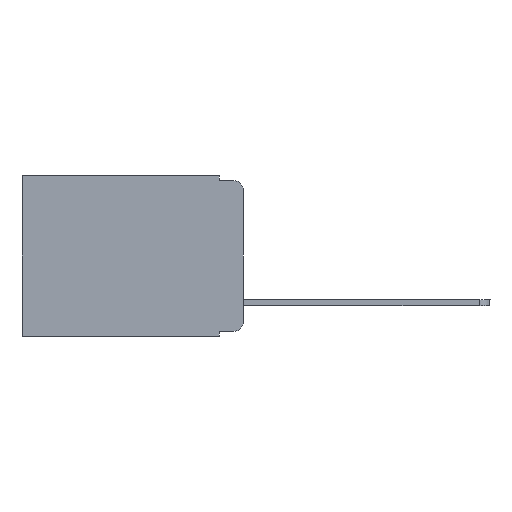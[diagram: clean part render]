
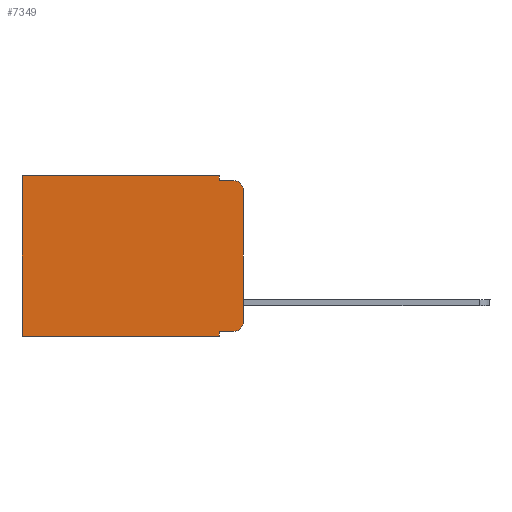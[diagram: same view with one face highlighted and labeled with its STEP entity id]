
A CAD part, left-side view. The second image highlights one B-rep face of the part: STEP entity #7349.
In plain terms, the highlighted planar face has unit normal (-1, 0, 0).
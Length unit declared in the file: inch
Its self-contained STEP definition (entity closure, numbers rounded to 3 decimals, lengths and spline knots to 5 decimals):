
#12 = EDGE_LOOP ( 'NONE', ( #2048, #13810, #19755, #18874, #17836, #16776, #1438, #20468, #11609, #22706 ) ) ;
#314 = AXIS2_PLACEMENT_3D ( 'NONE', #17217, #21081, #20713 ) ;
#598 = LINE ( 'NONE', #15646, #19737 ) ;
#1134 = VERTEX_POINT ( 'NONE', #3413 ) ;
#1438 = ORIENTED_EDGE ( 'NONE', *, *, #14756, .F. ) ;
#1525 = LINE ( 'NONE', #3345, #20152 ) ;
#1850 = VERTEX_POINT ( 'NONE', #20953 ) ;
#2048 = ORIENTED_EDGE ( 'NONE', *, *, #21662, .F. ) ;
#2523 = EDGE_CURVE ( 'NONE', #10159, #13411, #5478, .T. ) ;
#2542 = VERTEX_POINT ( 'NONE', #9267 ) ;
#3345 = CARTESIAN_POINT ( 'NONE',  ( 0.298, 0.051, 0. ) ) ;
#3413 = CARTESIAN_POINT ( 'NONE',  ( 0.298, 0.02, -0.333 ) ) ;
#3888 = DIRECTION ( 'NONE',  ( 0., 1., 0. ) ) ;
#4215 = FACE_OUTER_BOUND ( 'NONE', #12, .T. ) ;
#4271 = CARTESIAN_POINT ( 'NONE',  ( 0.298, 0., -0.03 ) ) ;
#4284 = DIRECTION ( 'NONE',  ( 0., -1., 0. ) ) ;
#4562 = DIRECTION ( 'NONE',  ( 0., 0., -1. ) ) ;
#5035 = DIRECTION ( 'NONE',  ( 0., 0., -1. ) ) ;
#5478 = LINE ( 'NONE', #5716, #11125 ) ;
#5716 = CARTESIAN_POINT ( 'NONE',  ( 0.298, 0., 0. ) ) ;
#5770 = VECTOR ( 'NONE', #23437, 39.37008 ) ;
#6905 = CARTESIAN_POINT ( 'NONE',  ( 0.298, 0.051, -0.01 ) ) ;
#7349 = ADVANCED_FACE ( 'NONE', ( #4215 ), #13361, .F. ) ;
#7800 = EDGE_CURVE ( 'NONE', #9199, #1134, #7839, .T. ) ;
#7839 = LINE ( 'NONE', #19101, #15271 ) ;
#8547 = CARTESIAN_POINT ( 'NONE',  ( 0.298, 0.02, -0.03 ) ) ;
#8747 = CARTESIAN_POINT ( 'NONE',  ( 0.298, 0.473, -0.343 ) ) ;
#8871 = VERTEX_POINT ( 'NONE', #16335 ) ;
#9199 = VERTEX_POINT ( 'NONE', #14371 ) ;
#9267 = CARTESIAN_POINT ( 'NONE',  ( 0.298, 0.051, -0.343 ) ) ;
#9456 = CARTESIAN_POINT ( 'NONE',  ( 0.298, 0.051, 0. ) ) ;
#10115 = EDGE_CURVE ( 'NONE', #1850, #12892, #16125, .T. ) ;
#10159 = VERTEX_POINT ( 'NONE', #9456 ) ;
#10241 = LINE ( 'NONE', #22938, #11379 ) ;
#10627 = DIRECTION ( 'NONE',  ( -1., 0., 0. ) ) ;
#10691 = DIRECTION ( 'NONE',  ( -1., 0., 0. ) ) ;
#11125 = VECTOR ( 'NONE', #3888, 39.37008 ) ;
#11379 = VECTOR ( 'NONE', #14103, 39.37008 ) ;
#11609 = ORIENTED_EDGE ( 'NONE', *, *, #7800, .T. ) ;
#11741 = AXIS2_PLACEMENT_3D ( 'NONE', #8547, #10627, #21252 ) ;
#12623 = DIRECTION ( 'NONE',  ( 0., -1., 0. ) ) ;
#12730 = VECTOR ( 'NONE', #12623, 39.37008 ) ;
#12798 = VECTOR ( 'NONE', #21095, 39.37008 ) ;
#12892 = VERTEX_POINT ( 'NONE', #22839 ) ;
#12999 = VERTEX_POINT ( 'NONE', #4271 ) ;
#13361 = PLANE ( 'NONE',  #314 ) ;
#13411 = VERTEX_POINT ( 'NONE', #20738 ) ;
#13734 = LINE ( 'NONE', #19397, #12798 ) ;
#13810 = ORIENTED_EDGE ( 'NONE', *, *, #14302, .T. ) ;
#14103 = DIRECTION ( 'NONE',  ( 0., 1., 0. ) ) ;
#14302 = EDGE_CURVE ( 'NONE', #12999, #12892, #22151, .T. ) ;
#14371 = CARTESIAN_POINT ( 'NONE',  ( 0.298, 0.051, -0.333 ) ) ;
#14756 = EDGE_CURVE ( 'NONE', #2542, #14995, #10241, .T. ) ;
#14881 = AXIS2_PLACEMENT_3D ( 'NONE', #19860, #10691, #18048 ) ;
#14995 = VERTEX_POINT ( 'NONE', #8747 ) ;
#15271 = VECTOR ( 'NONE', #4284, 39.37008 ) ;
#15646 = CARTESIAN_POINT ( 'NONE',  ( 0.298, 0.051, 0. ) ) ;
#15832 = LINE ( 'NONE', #17524, #5770 ) ;
#16125 = LINE ( 'NONE', #6905, #12730 ) ;
#16335 = CARTESIAN_POINT ( 'NONE',  ( 0.298, 0., -0.313 ) ) ;
#16776 = ORIENTED_EDGE ( 'NONE', *, *, #20930, .T. ) ;
#17217 = CARTESIAN_POINT ( 'NONE',  ( 0.298, 0., 0. ) ) ;
#17289 = EDGE_CURVE ( 'NONE', #1134, #8871, #18358, .T. ) ;
#17524 = CARTESIAN_POINT ( 'NONE',  ( 0.298, 0.473, 0. ) ) ;
#17836 = ORIENTED_EDGE ( 'NONE', *, *, #2523, .T. ) ;
#18048 = DIRECTION ( 'NONE',  ( 0., 0., -1. ) ) ;
#18358 = CIRCLE ( 'NONE', #14881, 0.02 ) ;
#18874 = ORIENTED_EDGE ( 'NONE', *, *, #22333, .F. ) ;
#19101 = CARTESIAN_POINT ( 'NONE',  ( 0.298, 0.051, -0.333 ) ) ;
#19397 = CARTESIAN_POINT ( 'NONE',  ( 0.298, 0., 0. ) ) ;
#19737 = VECTOR ( 'NONE', #4562, 39.37008 ) ;
#19755 = ORIENTED_EDGE ( 'NONE', *, *, #10115, .F. ) ;
#19860 = CARTESIAN_POINT ( 'NONE',  ( 0.298, 0.02, -0.313 ) ) ;
#20152 = VECTOR ( 'NONE', #5035, 39.37008 ) ;
#20468 = ORIENTED_EDGE ( 'NONE', *, *, #22144, .F. ) ;
#20713 = DIRECTION ( 'NONE',  ( 0., 0., -1. ) ) ;
#20738 = CARTESIAN_POINT ( 'NONE',  ( 0.298, 0.473, 0. ) ) ;
#20930 = EDGE_CURVE ( 'NONE', #13411, #14995, #15832, .T. ) ;
#20953 = CARTESIAN_POINT ( 'NONE',  ( 0.298, 0.051, -0.01 ) ) ;
#21081 = DIRECTION ( 'NONE',  ( 1., 0., 0. ) ) ;
#21095 = DIRECTION ( 'NONE',  ( 0., 0., -1. ) ) ;
#21252 = DIRECTION ( 'NONE',  ( 0., 0., -1. ) ) ;
#21662 = EDGE_CURVE ( 'NONE', #12999, #8871, #13734, .T. ) ;
#22144 = EDGE_CURVE ( 'NONE', #9199, #2542, #598, .T. ) ;
#22151 = CIRCLE ( 'NONE', #11741, 0.02 ) ;
#22333 = EDGE_CURVE ( 'NONE', #10159, #1850, #1525, .T. ) ;
#22706 = ORIENTED_EDGE ( 'NONE', *, *, #17289, .T. ) ;
#22839 = CARTESIAN_POINT ( 'NONE',  ( 0.298, 0.02, -0.01 ) ) ;
#22938 = CARTESIAN_POINT ( 'NONE',  ( 0.298, 0., -0.343 ) ) ;
#23437 = DIRECTION ( 'NONE',  ( 0., 0., -1. ) ) ;
